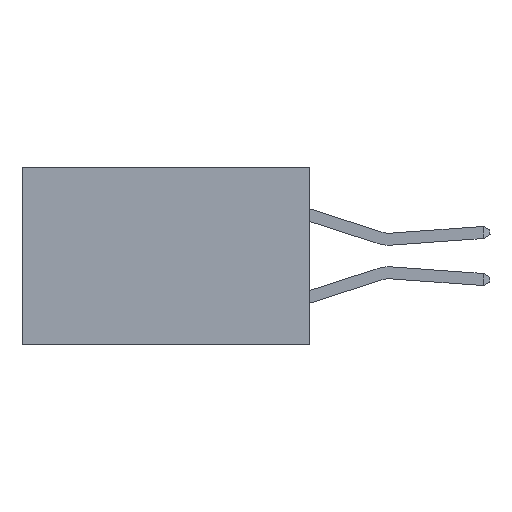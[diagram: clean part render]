
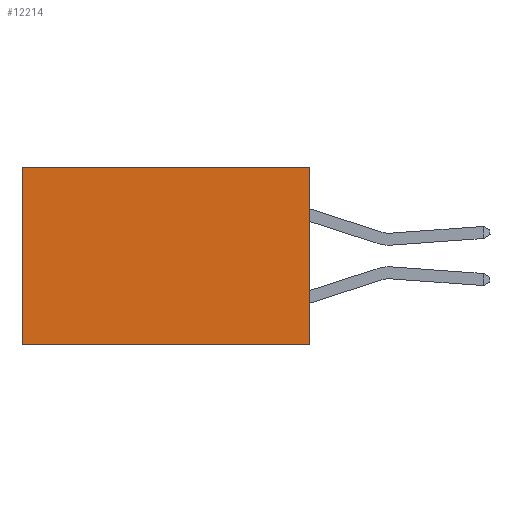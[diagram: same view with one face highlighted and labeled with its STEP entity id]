
A CAD part, left-side view. The second image highlights one B-rep face of the part: STEP entity #12214.
In plain terms, the highlighted planar face has unit normal (-1, 0, 0).
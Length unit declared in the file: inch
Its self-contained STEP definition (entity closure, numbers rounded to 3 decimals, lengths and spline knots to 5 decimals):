
#202 = EDGE_CURVE ( 'NONE', #7016, #19932, #15241, .T. ) ;
#328 = DIRECTION ( 'NONE',  ( 0., 0., -1. ) ) ;
#706 = DIRECTION ( 'NONE',  ( 0., 1., 0. ) ) ;
#1709 = EDGE_CURVE ( 'NONE', #19932, #5624, #12544, .T. ) ;
#2652 = AXIS2_PLACEMENT_3D ( 'NONE', #12818, #8181, #18899 ) ;
#3395 = PLANE ( 'NONE',  #2652 ) ;
#4036 = ORIENTED_EDGE ( 'NONE', *, *, #202, .T. ) ;
#4432 = DIRECTION ( 'NONE',  ( 0., 0., -1. ) ) ;
#5145 = CARTESIAN_POINT ( 'NONE',  ( 0.298, 0., 0. ) ) ;
#5624 = VERTEX_POINT ( 'NONE', #7311 ) ;
#5702 = CARTESIAN_POINT ( 'NONE',  ( 0.298, 0., -0.37 ) ) ;
#7016 = VERTEX_POINT ( 'NONE', #15710 ) ;
#7311 = CARTESIAN_POINT ( 'NONE',  ( 0.298, 0.6, -0.37 ) ) ;
#8181 = DIRECTION ( 'NONE',  ( 1., 0., 0. ) ) ;
#8199 = CARTESIAN_POINT ( 'NONE',  ( 0.298, 0.6, 0. ) ) ;
#8937 = ORIENTED_EDGE ( 'NONE', *, *, #18915, .F. ) ;
#9425 = ORIENTED_EDGE ( 'NONE', *, *, #1709, .T. ) ;
#10488 = VECTOR ( 'NONE', #328, 39.37008 ) ;
#10755 = VERTEX_POINT ( 'NONE', #17067 ) ;
#11414 = CARTESIAN_POINT ( 'NONE',  ( 0.298, 0., 0. ) ) ;
#12214 = ADVANCED_FACE ( 'NONE', ( #12234 ), #3395, .F. ) ;
#12234 = FACE_OUTER_BOUND ( 'NONE', #18576, .T. ) ;
#12544 = LINE ( 'NONE', #18535, #20086 ) ;
#12818 = CARTESIAN_POINT ( 'NONE',  ( 0.298, 0., 0. ) ) ;
#12985 = EDGE_CURVE ( 'NONE', #7016, #10755, #19995, .T. ) ;
#13509 = VECTOR ( 'NONE', #18041, 39.37008 ) ;
#15225 = LINE ( 'NONE', #5702, #13509 ) ;
#15241 = LINE ( 'NONE', #5145, #18750 ) ;
#15342 = ORIENTED_EDGE ( 'NONE', *, *, #12985, .F. ) ;
#15710 = CARTESIAN_POINT ( 'NONE',  ( 0.298, 0., 0. ) ) ;
#17067 = CARTESIAN_POINT ( 'NONE',  ( 0.298, 0., -0.37 ) ) ;
#18041 = DIRECTION ( 'NONE',  ( 0., 1., 0. ) ) ;
#18535 = CARTESIAN_POINT ( 'NONE',  ( 0.298, 0.6, 0. ) ) ;
#18576 = EDGE_LOOP ( 'NONE', ( #9425, #8937, #15342, #4036 ) ) ;
#18750 = VECTOR ( 'NONE', #706, 39.37008 ) ;
#18899 = DIRECTION ( 'NONE',  ( 0., 0., -1. ) ) ;
#18915 = EDGE_CURVE ( 'NONE', #10755, #5624, #15225, .T. ) ;
#19932 = VERTEX_POINT ( 'NONE', #8199 ) ;
#19995 = LINE ( 'NONE', #11414, #10488 ) ;
#20086 = VECTOR ( 'NONE', #4432, 39.37008 ) ;
